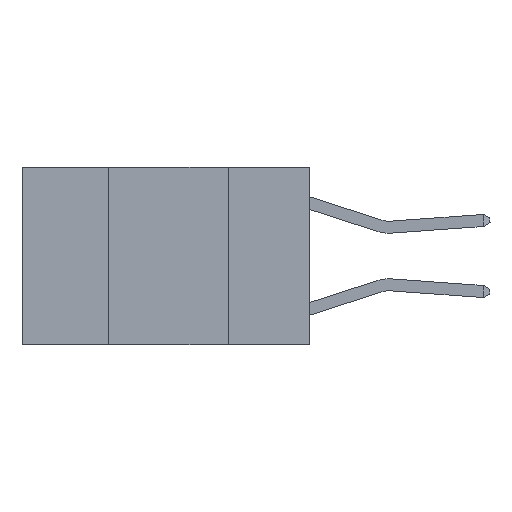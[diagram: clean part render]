
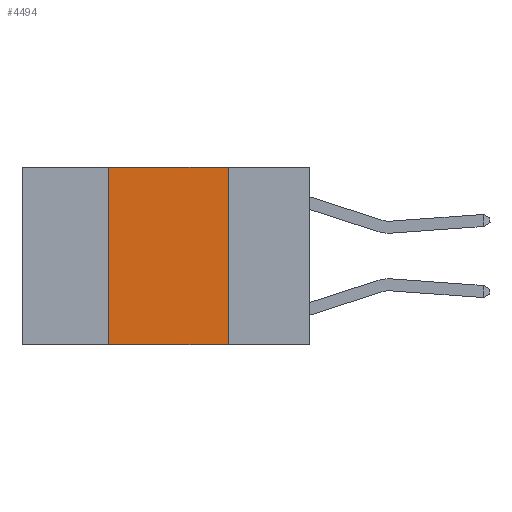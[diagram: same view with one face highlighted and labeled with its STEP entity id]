
A CAD part, left-side view. The second image highlights one B-rep face of the part: STEP entity #4494.
In plain terms, the highlighted planar face has unit normal (-1, 0, 0).
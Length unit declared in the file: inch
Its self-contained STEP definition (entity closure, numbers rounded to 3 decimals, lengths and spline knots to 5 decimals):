
#242 = AXIS2_PLACEMENT_3D ( 'NONE', #4846, #6997, #2725 ) ;
#437 = PLANE ( 'NONE',  #242 ) ;
#711 = CARTESIAN_POINT ( 'NONE',  ( 0., 0.42, -0.37 ) ) ;
#1142 = LINE ( 'NONE', #9290, #4581 ) ;
#1340 = VERTEX_POINT ( 'NONE', #711 ) ;
#1416 = ORIENTED_EDGE ( 'NONE', *, *, #8572, .F. ) ;
#1593 = VERTEX_POINT ( 'NONE', #4060 ) ;
#2201 = CARTESIAN_POINT ( 'NONE',  ( 0., 0.42, 0. ) ) ;
#2380 = ORIENTED_EDGE ( 'NONE', *, *, #6783, .F. ) ;
#2426 = VERTEX_POINT ( 'NONE', #7757 ) ;
#2674 = CARTESIAN_POINT ( 'NONE',  ( 0., 0.17, 0. ) ) ;
#2725 = DIRECTION ( 'NONE',  ( 0., 0., -1. ) ) ;
#2828 = CARTESIAN_POINT ( 'NONE',  ( 0., 0.42, 0. ) ) ;
#3012 = EDGE_LOOP ( 'NONE', ( #2380, #1416, #3810, #6582 ) ) ;
#3733 = VECTOR ( 'NONE', #4704, 39.37008 ) ;
#3810 = ORIENTED_EDGE ( 'NONE', *, *, #6319, .F. ) ;
#3941 = LINE ( 'NONE', #8181, #3733 ) ;
#4060 = CARTESIAN_POINT ( 'NONE',  ( 0., 0.17, -0.37 ) ) ;
#4494 = ADVANCED_FACE ( 'NONE', ( #8860 ), #437, .F. ) ;
#4581 = VECTOR ( 'NONE', #6572, 39.37008 ) ;
#4704 = DIRECTION ( 'NONE',  ( 0., -1., 0. ) ) ;
#4846 = CARTESIAN_POINT ( 'NONE',  ( 0., 0.6, 0. ) ) ;
#5379 = EDGE_CURVE ( 'NONE', #1340, #1593, #3941, .T. ) ;
#5841 = VECTOR ( 'NONE', #8503, 39.37008 ) ;
#6056 = LINE ( 'NONE', #2828, #5841 ) ;
#6260 = DIRECTION ( 'NONE',  ( 0., 0., -1. ) ) ;
#6283 = VECTOR ( 'NONE', #6260, 39.37008 ) ;
#6319 = EDGE_CURVE ( 'NONE', #1340, #7786, #6056, .T. ) ;
#6572 = DIRECTION ( 'NONE',  ( 0., -1., 0. ) ) ;
#6582 = ORIENTED_EDGE ( 'NONE', *, *, #5379, .T. ) ;
#6783 = EDGE_CURVE ( 'NONE', #2426, #1593, #8094, .T. ) ;
#6997 = DIRECTION ( 'NONE',  ( 1., 0., 0. ) ) ;
#7757 = CARTESIAN_POINT ( 'NONE',  ( 0., 0.17, 0. ) ) ;
#7786 = VERTEX_POINT ( 'NONE', #2201 ) ;
#8094 = LINE ( 'NONE', #2674, #6283 ) ;
#8181 = CARTESIAN_POINT ( 'NONE',  ( 0., 0.6, -0.37 ) ) ;
#8503 = DIRECTION ( 'NONE',  ( 0., 0., 1. ) ) ;
#8572 = EDGE_CURVE ( 'NONE', #7786, #2426, #1142, .T. ) ;
#8860 = FACE_OUTER_BOUND ( 'NONE', #3012, .T. ) ;
#9290 = CARTESIAN_POINT ( 'NONE',  ( 0., 0.6, 0. ) ) ;
